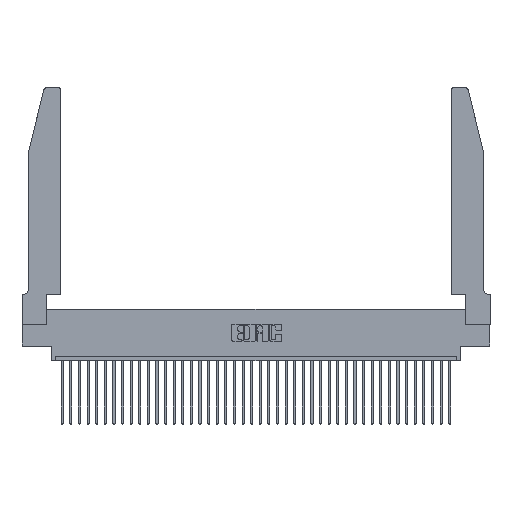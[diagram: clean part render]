
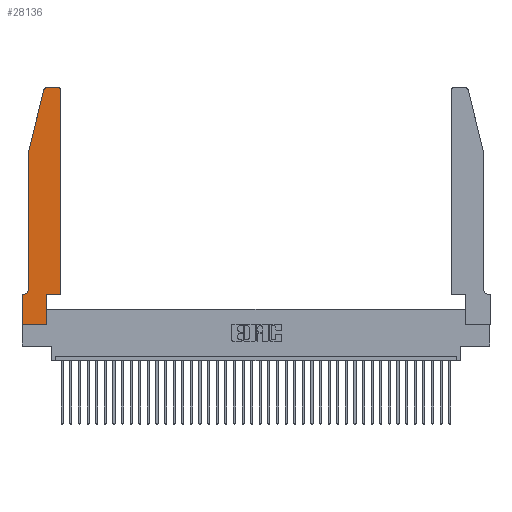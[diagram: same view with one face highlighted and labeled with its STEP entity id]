
A CAD part, top view. The second image highlights one B-rep face of the part: STEP entity #28136.
In plain terms, the highlighted planar face has unit normal (0, 0, 1).
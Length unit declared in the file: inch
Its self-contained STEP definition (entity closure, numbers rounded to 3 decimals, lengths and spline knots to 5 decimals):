
#42 = EDGE_LOOP ( 'NONE', ( #27494, #36349, #35796, #953, #30095, #9811, #2026, #18888, #15330, #34894, #13416, #29224 ) ) ;
#117 = CARTESIAN_POINT ( 'NONE',  ( 0.284, 2.75, 0.37 ) ) ;
#617 = LINE ( 'NONE', #27014, #27491 ) ;
#729 = LINE ( 'NONE', #23543, #8262 ) ;
#953 = ORIENTED_EDGE ( 'NONE', *, *, #19907, .T. ) ;
#1018 = EDGE_CURVE ( 'NONE', #21077, #1515, #35168, .T. ) ;
#1317 = DIRECTION ( 'NONE',  ( 1., 0., 0. ) ) ;
#1515 = VERTEX_POINT ( 'NONE', #2011 ) ;
#1674 = CARTESIAN_POINT ( 'NONE',  ( 0., 0., 0.37 ) ) ;
#1761 = DIRECTION ( 'NONE',  ( 1., 0., 0. ) ) ;
#2011 = CARTESIAN_POINT ( 'NONE',  ( 0., 0.35, 0.37 ) ) ;
#2026 = ORIENTED_EDGE ( 'NONE', *, *, #26111, .T. ) ;
#3074 = VERTEX_POINT ( 'NONE', #3166 ) ;
#3166 = CARTESIAN_POINT ( 'NONE',  ( 0.4205, 2.75, 0.37 ) ) ;
#3822 = AXIS2_PLACEMENT_3D ( 'NONE', #25809, #7746, #22332 ) ;
#4380 = VERTEX_POINT ( 'NONE', #117 ) ;
#6327 = CIRCLE ( 'NONE', #13446, 0.03 ) ;
#7227 = VERTEX_POINT ( 'NONE', #30345 ) ;
#7346 = VECTOR ( 'NONE', #26433, 39.37008 ) ;
#7426 = EDGE_CURVE ( 'NONE', #34194, #27323, #7802, .T. ) ;
#7488 = CIRCLE ( 'NONE', #3822, 0.07 ) ;
#7746 = DIRECTION ( 'NONE',  ( 0., 0., -1. ) ) ;
#7802 = LINE ( 'NONE', #20473, #7346 ) ;
#7804 = CARTESIAN_POINT ( 'NONE',  ( 0.2605, 2.75, 0.37 ) ) ;
#7823 = DIRECTION ( 'NONE',  ( 0., 0., 1. ) ) ;
#7953 = DIRECTION ( 'NONE',  ( 0., -1., 0. ) ) ;
#8262 = VECTOR ( 'NONE', #20644, 39.37008 ) ;
#8651 = CARTESIAN_POINT ( 'NONE',  ( 0.0755, 0.42, 0.37 ) ) ;
#9052 = DIRECTION ( 'NONE',  ( 0., 0., 1. ) ) ;
#9730 = DIRECTION ( 'NONE',  ( -1., 0., 0. ) ) ;
#9811 = ORIENTED_EDGE ( 'NONE', *, *, #1018, .T. ) ;
#10544 = CIRCLE ( 'NONE', #28869, 0.03 ) ;
#10687 = CARTESIAN_POINT ( 'NONE',  ( 0.4505, 0.35, 0.37 ) ) ;
#13137 = DIRECTION ( 'NONE',  ( 0., 0., 1. ) ) ;
#13363 = VERTEX_POINT ( 'NONE', #21718 ) ;
#13416 = ORIENTED_EDGE ( 'NONE', *, *, #35801, .T. ) ;
#13446 = AXIS2_PLACEMENT_3D ( 'NONE', #19688, #7823, #22282 ) ;
#15328 = CARTESIAN_POINT ( 'NONE',  ( 0., 0., 0.37 ) ) ;
#15330 = ORIENTED_EDGE ( 'NONE', *, *, #35946, .T. ) ;
#15652 = PLANE ( 'NONE',  #37094 ) ;
#15833 = CARTESIAN_POINT ( 'NONE',  ( 0.2865, 0., 0.37 ) ) ;
#17444 = FACE_OUTER_BOUND ( 'NONE', #42, .T. ) ;
#17492 = CARTESIAN_POINT ( 'NONE',  ( 0.2865, 0.35, 0.37 ) ) ;
#18496 = CARTESIAN_POINT ( 'NONE',  ( 0.4505, 2.72, 0.37 ) ) ;
#18548 = CARTESIAN_POINT ( 'NONE',  ( 0., 0.35, 0.37 ) ) ;
#18595 = DIRECTION ( 'NONE',  ( 0., -1., 0. ) ) ;
#18767 = EDGE_CURVE ( 'NONE', #4380, #7227, #10544, .T. ) ;
#18888 = ORIENTED_EDGE ( 'NONE', *, *, #7426, .T. ) ;
#19688 = CARTESIAN_POINT ( 'NONE',  ( 0.4205, 2.72, 0.37 ) ) ;
#19907 = EDGE_CURVE ( 'NONE', #13363, #35903, #21270, .T. ) ;
#20473 = CARTESIAN_POINT ( 'NONE',  ( 0., 0., 0.37 ) ) ;
#20558 = DIRECTION ( 'NONE',  ( -0.239, -0.971, 0. ) ) ;
#20644 = DIRECTION ( 'NONE',  ( 0., 1., 0. ) ) ;
#21055 = EDGE_CURVE ( 'NONE', #25153, #21177, #23136, .T. ) ;
#21077 = VERTEX_POINT ( 'NONE', #32174 ) ;
#21177 = VERTEX_POINT ( 'NONE', #24462 ) ;
#21270 = LINE ( 'NONE', #28554, #33522 ) ;
#21438 = CARTESIAN_POINT ( 'NONE',  ( 0.0755, 0.35, 0.37 ) ) ;
#21718 = CARTESIAN_POINT ( 'NONE',  ( 0.0755, 2., 0.37 ) ) ;
#22084 = VECTOR ( 'NONE', #9730, 39.37008 ) ;
#22282 = DIRECTION ( 'NONE',  ( 1., 0., 0. ) ) ;
#22332 = DIRECTION ( 'NONE',  ( -1., 0., 0. ) ) ;
#22603 = LINE ( 'NONE', #7804, #22084 ) ;
#23136 = LINE ( 'NONE', #10687, #23630 ) ;
#23543 = CARTESIAN_POINT ( 'NONE',  ( 0.2865, 0.35, 0.37 ) ) ;
#23630 = VECTOR ( 'NONE', #1761, 39.37008 ) ;
#24462 = CARTESIAN_POINT ( 'NONE',  ( 0.4505, 0.35, 0.37 ) ) ;
#25153 = VERTEX_POINT ( 'NONE', #17492 ) ;
#25671 = LINE ( 'NONE', #1674, #30806 ) ;
#25794 = DIRECTION ( 'NONE',  ( 0., 1., 0. ) ) ;
#25809 = CARTESIAN_POINT ( 'NONE',  ( 0.0055, 0.42, 0.37 ) ) ;
#26111 = EDGE_CURVE ( 'NONE', #1515, #34194, #25671, .T. ) ;
#26191 = VERTEX_POINT ( 'NONE', #18496 ) ;
#26242 = VECTOR ( 'NONE', #31097, 39.37008 ) ;
#26286 = EDGE_CURVE ( 'NONE', #7227, #13363, #617, .T. ) ;
#26433 = DIRECTION ( 'NONE',  ( 1., 0., 0. ) ) ;
#26615 = DIRECTION ( 'NONE',  ( 1., 0., 0. ) ) ;
#27014 = CARTESIAN_POINT ( 'NONE',  ( 0.0755, 2., 0.37 ) ) ;
#27323 = VERTEX_POINT ( 'NONE', #15833 ) ;
#27491 = VECTOR ( 'NONE', #20558, 39.37008 ) ;
#27494 = ORIENTED_EDGE ( 'NONE', *, *, #28340, .T. ) ;
#28136 = ADVANCED_FACE ( 'NONE', ( #17444 ), #15652, .T. ) ;
#28340 = EDGE_CURVE ( 'NONE', #3074, #4380, #22603, .T. ) ;
#28554 = CARTESIAN_POINT ( 'NONE',  ( 0.0755, 2., 0.37 ) ) ;
#28869 = AXIS2_PLACEMENT_3D ( 'NONE', #31348, #9052, #26615 ) ;
#29224 = ORIENTED_EDGE ( 'NONE', *, *, #36304, .T. ) ;
#29517 = VECTOR ( 'NONE', #25794, 39.37008 ) ;
#29592 = EDGE_CURVE ( 'NONE', #35903, #21077, #7488, .T. ) ;
#30095 = ORIENTED_EDGE ( 'NONE', *, *, #29592, .T. ) ;
#30345 = CARTESIAN_POINT ( 'NONE',  ( 0.25487, 2.72718, 0.37 ) ) ;
#30396 = LINE ( 'NONE', #37327, #29517 ) ;
#30806 = VECTOR ( 'NONE', #7953, 39.37008 ) ;
#31097 = DIRECTION ( 'NONE',  ( -1., 0., 0. ) ) ;
#31348 = CARTESIAN_POINT ( 'NONE',  ( 0.284, 2.72, 0.37 ) ) ;
#32174 = CARTESIAN_POINT ( 'NONE',  ( 0.0055, 0.35, 0.37 ) ) ;
#33522 = VECTOR ( 'NONE', #18595, 39.37008 ) ;
#34194 = VERTEX_POINT ( 'NONE', #15328 ) ;
#34894 = ORIENTED_EDGE ( 'NONE', *, *, #21055, .T. ) ;
#35168 = LINE ( 'NONE', #21438, #26242 ) ;
#35796 = ORIENTED_EDGE ( 'NONE', *, *, #26286, .T. ) ;
#35801 = EDGE_CURVE ( 'NONE', #21177, #26191, #30396, .T. ) ;
#35903 = VERTEX_POINT ( 'NONE', #8651 ) ;
#35946 = EDGE_CURVE ( 'NONE', #27323, #25153, #729, .T. ) ;
#36304 = EDGE_CURVE ( 'NONE', #26191, #3074, #6327, .T. ) ;
#36349 = ORIENTED_EDGE ( 'NONE', *, *, #18767, .T. ) ;
#37094 = AXIS2_PLACEMENT_3D ( 'NONE', #18548, #13137, #1317 ) ;
#37327 = CARTESIAN_POINT ( 'NONE',  ( 0.4505, 0.35, 0.37 ) ) ;
